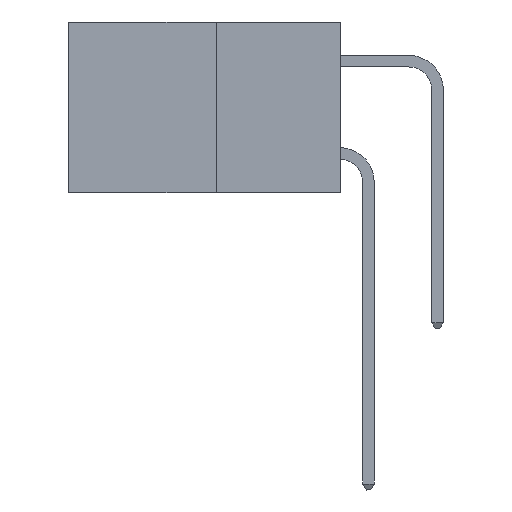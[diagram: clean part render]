
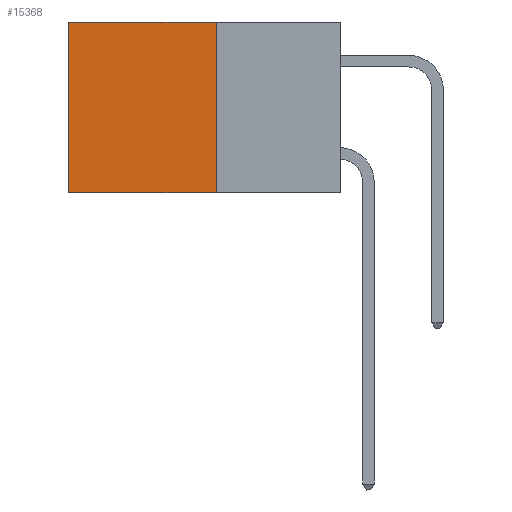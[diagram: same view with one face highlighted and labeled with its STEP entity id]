
A CAD part, left-side view. The second image highlights one B-rep face of the part: STEP entity #15368.
In plain terms, the highlighted planar face has unit normal (-1, 0, 0).
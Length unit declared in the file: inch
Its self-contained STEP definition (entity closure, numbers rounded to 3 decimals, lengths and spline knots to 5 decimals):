
#526 = ORIENTED_EDGE ( 'NONE', *, *, #1180, .F. ) ;
#554 = DIRECTION ( 'NONE',  ( 0., 0., -1. ) ) ;
#1052 = DIRECTION ( 'NONE',  ( 0., 1., 0. ) ) ;
#1180 = EDGE_CURVE ( 'NONE', #11922, #11483, #4541, .T. ) ;
#1282 = VECTOR ( 'NONE', #554, 39.37008 ) ;
#2072 = VECTOR ( 'NONE', #1052, 39.37008 ) ;
#2614 = DIRECTION ( 'NONE',  ( 0., 1., 0. ) ) ;
#2835 = VERTEX_POINT ( 'NONE', #9883 ) ;
#3240 = LINE ( 'NONE', #13743, #2072 ) ;
#3274 = PLANE ( 'NONE',  #13541 ) ;
#3429 = EDGE_CURVE ( 'NONE', #4895, #2835, #3240, .T. ) ;
#4460 = DIRECTION ( 'NONE',  ( 0., 0., -1. ) ) ;
#4541 = LINE ( 'NONE', #11553, #13638 ) ;
#4875 = LINE ( 'NONE', #6565, #1282 ) ;
#4895 = VERTEX_POINT ( 'NONE', #10253 ) ;
#5776 = FACE_OUTER_BOUND ( 'NONE', #5780, .T. ) ;
#5780 = EDGE_LOOP ( 'NONE', ( #11505, #526, #6916, #15426 ) ) ;
#6565 = CARTESIAN_POINT ( 'NONE',  ( 0.277, 0.27, -0.37 ) ) ;
#6916 = ORIENTED_EDGE ( 'NONE', *, *, #15207, .F. ) ;
#8514 = CARTESIAN_POINT ( 'NONE',  ( 0.277, 0.59, -0.37 ) ) ;
#9883 = CARTESIAN_POINT ( 'NONE',  ( 0.277, 0.59, 0. ) ) ;
#10253 = CARTESIAN_POINT ( 'NONE',  ( 0.277, 0.27, 0. ) ) ;
#10309 = CARTESIAN_POINT ( 'NONE',  ( 0.277, 0.27, -0.37 ) ) ;
#10544 = CARTESIAN_POINT ( 'NONE',  ( 0.277, 0.59, -0.37 ) ) ;
#10599 = DIRECTION ( 'NONE',  ( 0., 0., -1. ) ) ;
#10952 = VECTOR ( 'NONE', #10599, 39.37008 ) ;
#11483 = VERTEX_POINT ( 'NONE', #8514 ) ;
#11505 = ORIENTED_EDGE ( 'NONE', *, *, #13283, .T. ) ;
#11553 = CARTESIAN_POINT ( 'NONE',  ( 0.277, 0.27, -0.37 ) ) ;
#11584 = DIRECTION ( 'NONE',  ( 1., 0., 0. ) ) ;
#11922 = VERTEX_POINT ( 'NONE', #15137 ) ;
#13283 = EDGE_CURVE ( 'NONE', #2835, #11483, #14080, .T. ) ;
#13541 = AXIS2_PLACEMENT_3D ( 'NONE', #10309, #11584, #4460 ) ;
#13638 = VECTOR ( 'NONE', #2614, 39.37008 ) ;
#13743 = CARTESIAN_POINT ( 'NONE',  ( 0.277, 0.27, 0. ) ) ;
#14080 = LINE ( 'NONE', #10544, #10952 ) ;
#15137 = CARTESIAN_POINT ( 'NONE',  ( 0.277, 0.27, -0.37 ) ) ;
#15207 = EDGE_CURVE ( 'NONE', #4895, #11922, #4875, .T. ) ;
#15368 = ADVANCED_FACE ( 'NONE', ( #5776 ), #3274, .F. ) ;
#15426 = ORIENTED_EDGE ( 'NONE', *, *, #3429, .T. ) ;
